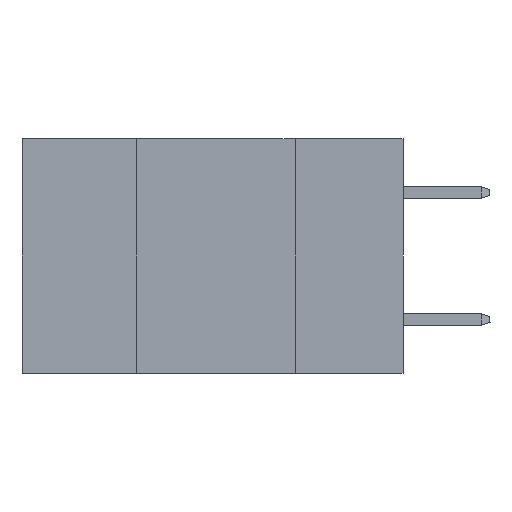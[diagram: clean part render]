
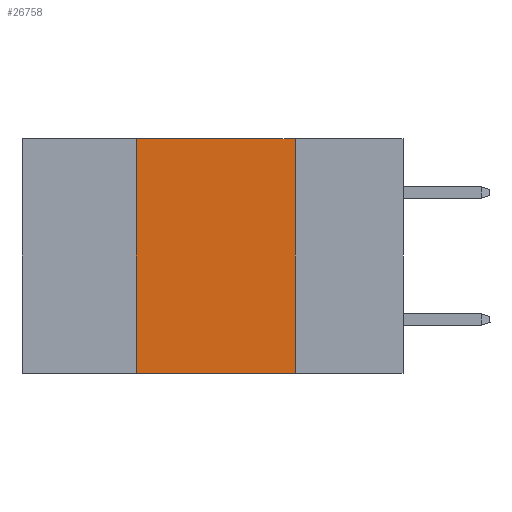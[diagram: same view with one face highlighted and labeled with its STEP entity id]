
A CAD part, left-side view. The second image highlights one B-rep face of the part: STEP entity #26758.
In plain terms, the highlighted planar face has unit normal (-1, 0, 0).
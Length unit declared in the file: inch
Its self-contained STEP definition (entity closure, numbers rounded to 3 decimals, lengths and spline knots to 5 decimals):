
#124 = CARTESIAN_POINT ( 'NONE',  ( 0., 0.6, 0. ) ) ;
#1755 = CARTESIAN_POINT ( 'NONE',  ( 0., 0.17, 0. ) ) ;
#2652 = VECTOR ( 'NONE', #16040, 39.37008 ) ;
#3585 = VECTOR ( 'NONE', #24384, 39.37008 ) ;
#3673 = CARTESIAN_POINT ( 'NONE',  ( 0., 0.6, 0. ) ) ;
#4669 = EDGE_CURVE ( 'NONE', #14174, #5014, #18115, .T. ) ;
#5014 = VERTEX_POINT ( 'NONE', #10667 ) ;
#8085 = ORIENTED_EDGE ( 'NONE', *, *, #17162, .F. ) ;
#8844 = PLANE ( 'NONE',  #24709 ) ;
#9131 = FACE_OUTER_BOUND ( 'NONE', #23432, .T. ) ;
#10278 = ORIENTED_EDGE ( 'NONE', *, *, #12456, .F. ) ;
#10657 = CARTESIAN_POINT ( 'NONE',  ( 0., 0.6, -0.37 ) ) ;
#10667 = CARTESIAN_POINT ( 'NONE',  ( 0., 0.17, -0.37 ) ) ;
#10668 = EDGE_CURVE ( 'NONE', #28011, #5014, #15104, .T. ) ;
#11065 = DIRECTION ( 'NONE',  ( 0., -1., 0. ) ) ;
#12456 = EDGE_CURVE ( 'NONE', #28011, #18407, #26896, .T. ) ;
#12724 = VECTOR ( 'NONE', #11065, 39.37008 ) ;
#13167 = DIRECTION ( 'NONE',  ( 0., -1., 0. ) ) ;
#13419 = DIRECTION ( 'NONE',  ( 1., 0., 0. ) ) ;
#14174 = VERTEX_POINT ( 'NONE', #1755 ) ;
#14471 = VECTOR ( 'NONE', #13167, 39.37008 ) ;
#15104 = LINE ( 'NONE', #10657, #14471 ) ;
#16040 = DIRECTION ( 'NONE',  ( 0., 0., -1. ) ) ;
#16311 = ORIENTED_EDGE ( 'NONE', *, *, #4669, .F. ) ;
#16327 = CARTESIAN_POINT ( 'NONE',  ( 0., 0.17, 0. ) ) ;
#17162 = EDGE_CURVE ( 'NONE', #18407, #14174, #19777, .T. ) ;
#18115 = LINE ( 'NONE', #16327, #2652 ) ;
#18407 = VERTEX_POINT ( 'NONE', #21137 ) ;
#19777 = LINE ( 'NONE', #3673, #12724 ) ;
#19907 = DIRECTION ( 'NONE',  ( 0., 0., -1. ) ) ;
#20096 = CARTESIAN_POINT ( 'NONE',  ( 0., 0.42, 0. ) ) ;
#21137 = CARTESIAN_POINT ( 'NONE',  ( 0., 0.42, 0. ) ) ;
#22416 = CARTESIAN_POINT ( 'NONE',  ( 0., 0.42, -0.37 ) ) ;
#23432 = EDGE_LOOP ( 'NONE', ( #16311, #8085, #10278, #28327 ) ) ;
#24384 = DIRECTION ( 'NONE',  ( 0., 0., 1. ) ) ;
#24709 = AXIS2_PLACEMENT_3D ( 'NONE', #124, #13419, #19907 ) ;
#26758 = ADVANCED_FACE ( 'NONE', ( #9131 ), #8844, .F. ) ;
#26896 = LINE ( 'NONE', #20096, #3585 ) ;
#28011 = VERTEX_POINT ( 'NONE', #22416 ) ;
#28327 = ORIENTED_EDGE ( 'NONE', *, *, #10668, .T. ) ;
